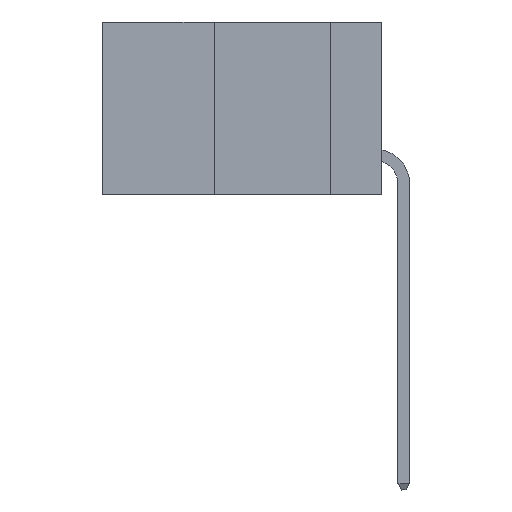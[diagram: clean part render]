
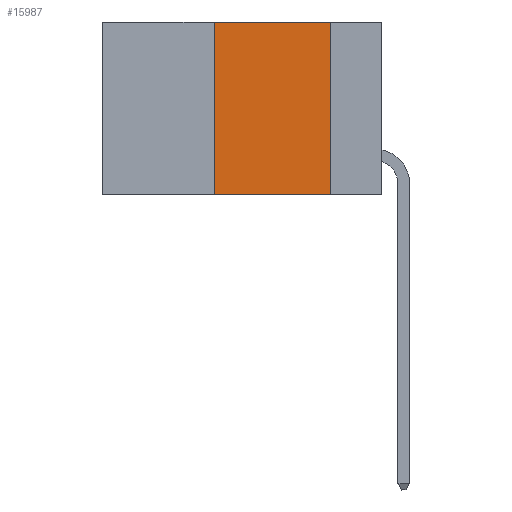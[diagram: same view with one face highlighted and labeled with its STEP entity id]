
A CAD part, left-side view. The second image highlights one B-rep face of the part: STEP entity #15987.
In plain terms, the highlighted planar face has unit normal (-1, 0, 0).
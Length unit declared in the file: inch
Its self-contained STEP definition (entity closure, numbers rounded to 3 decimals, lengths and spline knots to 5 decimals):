
#775 = FACE_OUTER_BOUND ( 'NONE', #9513, .T. ) ;
#3171 = AXIS2_PLACEMENT_3D ( 'NONE', #32294, #39875, #16729 ) ;
#3524 = DIRECTION ( 'NONE',  ( 0., 0., -1. ) ) ;
#5453 = CARTESIAN_POINT ( 'NONE',  ( 0., 0.36, -0.37 ) ) ;
#5559 = CARTESIAN_POINT ( 'NONE',  ( 0., 0.6, -0.37 ) ) ;
#6056 = LINE ( 'NONE', #41202, #42847 ) ;
#7432 = EDGE_CURVE ( 'NONE', #46050, #13083, #6056, .T. ) ;
#8066 = ORIENTED_EDGE ( 'NONE', *, *, #12260, .F. ) ;
#8463 = CARTESIAN_POINT ( 'NONE',  ( 0., 0.11, -0.37 ) ) ;
#9513 = EDGE_LOOP ( 'NONE', ( #27248, #18375, #8066, #13477 ) ) ;
#10771 = DIRECTION ( 'NONE',  ( 0., -1., 0. ) ) ;
#12260 = EDGE_CURVE ( 'NONE', #38145, #25917, #48752, .T. ) ;
#13083 = VERTEX_POINT ( 'NONE', #8463 ) ;
#13477 = ORIENTED_EDGE ( 'NONE', *, *, #30607, .T. ) ;
#14401 = CARTESIAN_POINT ( 'NONE',  ( 0., 0.36, 0. ) ) ;
#14471 = CARTESIAN_POINT ( 'NONE',  ( 0., 0.6, 0. ) ) ;
#15987 = ADVANCED_FACE ( 'NONE', ( #775 ), #17066, .F. ) ;
#16729 = DIRECTION ( 'NONE',  ( 0., 0., -1. ) ) ;
#17066 = PLANE ( 'NONE',  #3171 ) ;
#18375 = ORIENTED_EDGE ( 'NONE', *, *, #20608, .F. ) ;
#18401 = LINE ( 'NONE', #14471, #43260 ) ;
#20608 = EDGE_CURVE ( 'NONE', #25917, #46050, #18401, .T. ) ;
#22141 = LINE ( 'NONE', #5559, #42239 ) ;
#25396 = DIRECTION ( 'NONE',  ( 0., 0., 1. ) ) ;
#25917 = VERTEX_POINT ( 'NONE', #14401 ) ;
#27248 = ORIENTED_EDGE ( 'NONE', *, *, #7432, .F. ) ;
#29417 = CARTESIAN_POINT ( 'NONE',  ( 0., 0.11, 0. ) ) ;
#30607 = EDGE_CURVE ( 'NONE', #38145, #13083, #22141, .T. ) ;
#32120 = DIRECTION ( 'NONE',  ( 0., -1., 0. ) ) ;
#32294 = CARTESIAN_POINT ( 'NONE',  ( 0., 0.6, 0. ) ) ;
#38145 = VERTEX_POINT ( 'NONE', #5453 ) ;
#38617 = VECTOR ( 'NONE', #25396, 39.37008 ) ;
#39875 = DIRECTION ( 'NONE',  ( 1., 0., 0. ) ) ;
#39917 = CARTESIAN_POINT ( 'NONE',  ( 0., 0.36, 0. ) ) ;
#41202 = CARTESIAN_POINT ( 'NONE',  ( 0., 0.11, 0. ) ) ;
#42239 = VECTOR ( 'NONE', #32120, 39.37008 ) ;
#42847 = VECTOR ( 'NONE', #3524, 39.37008 ) ;
#43260 = VECTOR ( 'NONE', #10771, 39.37008 ) ;
#46050 = VERTEX_POINT ( 'NONE', #29417 ) ;
#48752 = LINE ( 'NONE', #39917, #38617 ) ;
